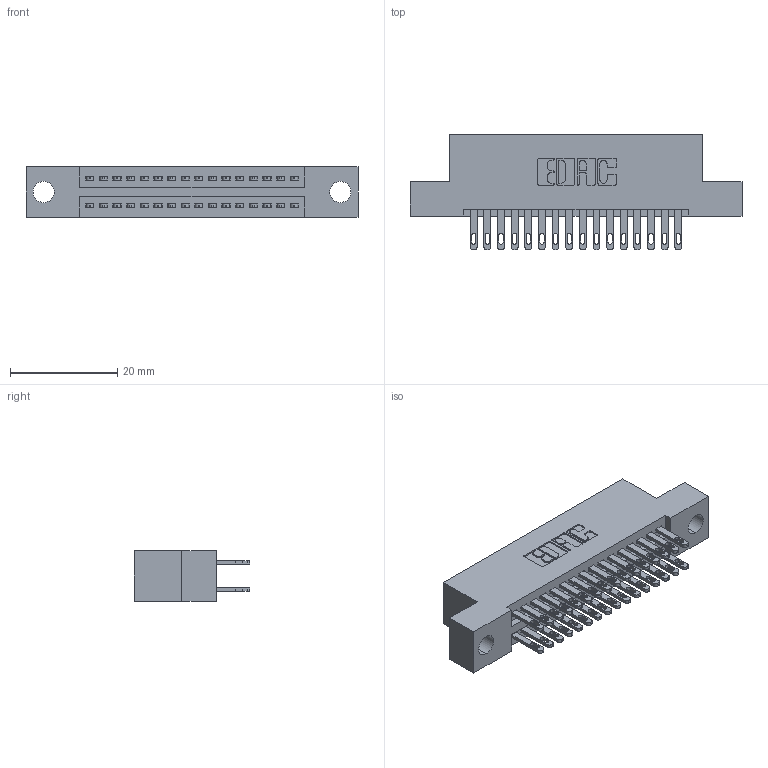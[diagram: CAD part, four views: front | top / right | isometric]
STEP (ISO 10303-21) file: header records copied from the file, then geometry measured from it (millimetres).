
FILE_DESCRIPTION (( 'STEP AP203' ), '1' );
FILE_NAME ('345-032-500-204.STEP', '2021-05-19T23:35:05', ( '' ), ( '' ), 'SwSTEP 2.0', 'SolidWorks 2020', '' );
FILE_SCHEMA (( 'CONFIG_CONTROL_DESIGN' ));
Length unit declared in the file: inch
Products named in the file (3): 345-292-001_345-293-100; 345-032-500-204; 345 Part_Flush Mounting Lugs - 0.156 Dia-TI
Assembly tree (33 placements, depth 2):
  345-032-500-204
    345 Part_Flush Mounting Lugs - 0.156 Dia-TI
    345-292-001_345-293-100  x32
Bounding box: 61.85 x 21.51 x 9.4 mm (x, y, z)
Volume: 5758.6 mm3; surface area: 8186.5 mm2
Topology: 33 solids, 33 shells, 1612 faces, 4889 edges, 3258 vertices
Faces by surface type: plane 958, cylinder 654
Entity records: 16403 total; most frequent: CARTESIAN_POINT 2778, ORIENTED_EDGE 2710, DIRECTION 2483, EDGE_CURVE 1355, VECTOR 1155, LINE 1155, VERTEX_POINT 902, AXIS2_PLACEMENT_3D 664
